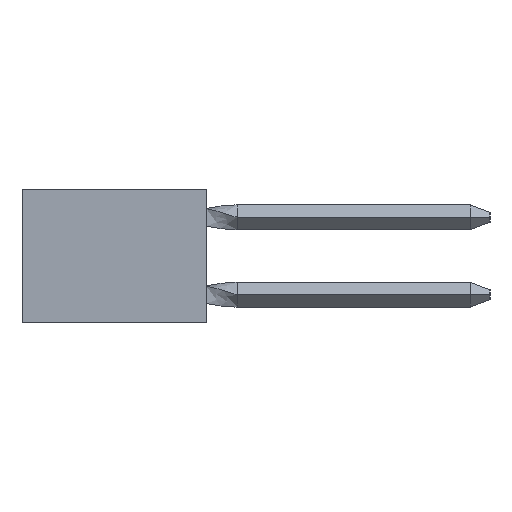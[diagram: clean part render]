
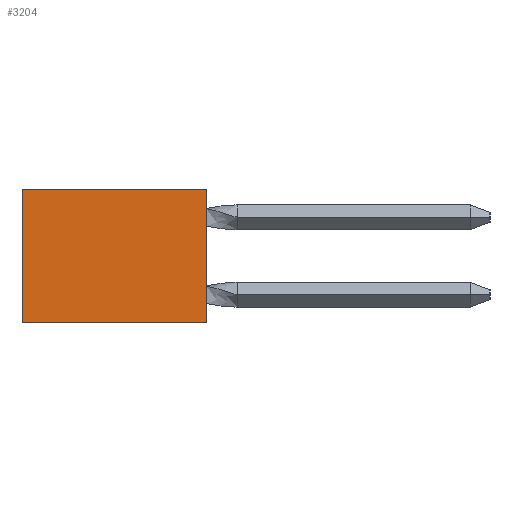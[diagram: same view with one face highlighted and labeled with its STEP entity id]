
A CAD part, left-side view. The second image highlights one B-rep face of the part: STEP entity #3204.
In plain terms, the highlighted planar face has unit normal (-1, 0, 0).
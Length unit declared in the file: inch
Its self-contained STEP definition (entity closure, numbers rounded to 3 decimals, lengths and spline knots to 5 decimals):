
#150 = VERTEX_POINT ( 'NONE', #936 ) ;
#936 = CARTESIAN_POINT ( 'NONE',  ( 0.298, 0.473, 0. ) ) ;
#1374 = PLANE ( 'NONE',  #10761 ) ;
#1959 = DIRECTION ( 'NONE',  ( 0., 1., 0. ) ) ;
#2646 = LINE ( 'NONE', #5965, #28777 ) ;
#3204 = ADVANCED_FACE ( 'NONE', ( #22564 ), #1374, .F. ) ;
#3573 = LINE ( 'NONE', #21360, #28144 ) ;
#5477 = LINE ( 'NONE', #7604, #5864 ) ;
#5864 = VECTOR ( 'NONE', #19530, 39.37008 ) ;
#5965 = CARTESIAN_POINT ( 'NONE',  ( 0.298, 0.473, -0.343 ) ) ;
#6418 = DIRECTION ( 'NONE',  ( 0., 1., 0. ) ) ;
#7604 = CARTESIAN_POINT ( 'NONE',  ( 0.298, 0., -0.343 ) ) ;
#8660 = EDGE_CURVE ( 'NONE', #9651, #150, #3573, .T. ) ;
#9651 = VERTEX_POINT ( 'NONE', #29059 ) ;
#9727 = EDGE_CURVE ( 'NONE', #29435, #9651, #5477, .T. ) ;
#10743 = CARTESIAN_POINT ( 'NONE',  ( 0.298, 0.473, 0. ) ) ;
#10747 = ORIENTED_EDGE ( 'NONE', *, *, #8660, .T. ) ;
#10761 = AXIS2_PLACEMENT_3D ( 'NONE', #10847, #30500, #20829 ) ;
#10847 = CARTESIAN_POINT ( 'NONE',  ( 0.298, -0.027, 0. ) ) ;
#11430 = EDGE_CURVE ( 'NONE', #29435, #24690, #2646, .T. ) ;
#12585 = VECTOR ( 'NONE', #15784, 39.37008 ) ;
#14485 = ORIENTED_EDGE ( 'NONE', *, *, #26614, .T. ) ;
#15784 = DIRECTION ( 'NONE',  ( 0., 0., -1. ) ) ;
#15908 = CARTESIAN_POINT ( 'NONE',  ( 0.298, 0., -0.343 ) ) ;
#17198 = LINE ( 'NONE', #10743, #12585 ) ;
#17651 = ORIENTED_EDGE ( 'NONE', *, *, #9727, .T. ) ;
#19530 = DIRECTION ( 'NONE',  ( 0., 0., 1. ) ) ;
#20829 = DIRECTION ( 'NONE',  ( 0., 0., -1. ) ) ;
#21360 = CARTESIAN_POINT ( 'NONE',  ( 0.298, -0.027, 0. ) ) ;
#22564 = FACE_OUTER_BOUND ( 'NONE', #27463, .T. ) ;
#24690 = VERTEX_POINT ( 'NONE', #31792 ) ;
#26614 = EDGE_CURVE ( 'NONE', #150, #24690, #17198, .T. ) ;
#27310 = ORIENTED_EDGE ( 'NONE', *, *, #11430, .F. ) ;
#27463 = EDGE_LOOP ( 'NONE', ( #17651, #10747, #14485, #27310 ) ) ;
#28144 = VECTOR ( 'NONE', #6418, 39.37008 ) ;
#28777 = VECTOR ( 'NONE', #1959, 39.37008 ) ;
#29059 = CARTESIAN_POINT ( 'NONE',  ( 0.298, 0., 0. ) ) ;
#29435 = VERTEX_POINT ( 'NONE', #15908 ) ;
#30500 = DIRECTION ( 'NONE',  ( 1., 0., 0. ) ) ;
#31792 = CARTESIAN_POINT ( 'NONE',  ( 0.298, 0.473, -0.343 ) ) ;
